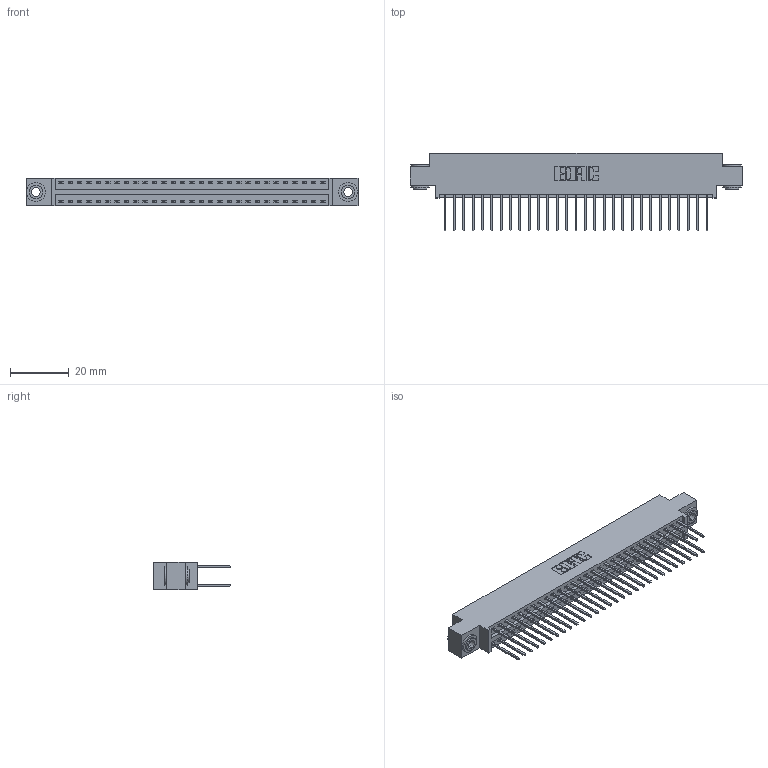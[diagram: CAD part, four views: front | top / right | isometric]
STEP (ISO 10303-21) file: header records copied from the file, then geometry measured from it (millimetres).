
FILE_DESCRIPTION (( 'STEP AP203' ), '1' );
FILE_NAME ('346-058-522-803.STEP', '2022-05-21T08:04:33', ( '' ), ( '' ), 'SwSTEP 2.0', 'SolidWorks 2020', '' );
FILE_SCHEMA (( 'CONFIG_CONTROL_DESIGN' ));
Length unit declared in the file: inch
Products named in the file (4): 346-058-522-803; 345-292-001_345-293-122; 345-250-002_345-250-002-102; 346 Part_0.170 Offset - 0.156 Dia-TH
Assembly tree (61 placements, depth 2):
  346-058-522-803
    346 Part_0.170 Offset - 0.156 Dia-TH
    345-292-001_345-293-122  x58
    345-250-002_345-250-002-102  x2
Bounding box: 112.65 x 26.42 x 9.4 mm (x, y, z)
Volume: 10879 mm3; surface area: 15866.9 mm2
Topology: 61 solids, 61 shells, 3194 faces, 9443 edges, 6214 vertices
Faces by surface type: plane 2134, cylinder 1052, cone 8
Entity records: 21892 total; most frequent: CARTESIAN_POINT 3609, ORIENTED_EDGE 3534, DIRECTION 3261, EDGE_CURVE 1767, LINE 1495, VECTOR 1495, VERTEX_POINT 1174, AXIS2_PLACEMENT_3D 883
